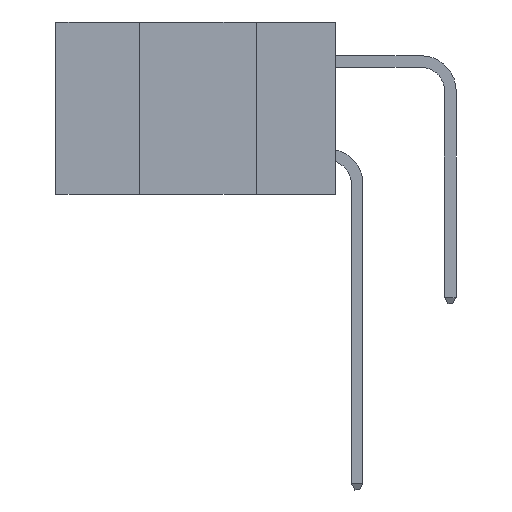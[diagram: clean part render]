
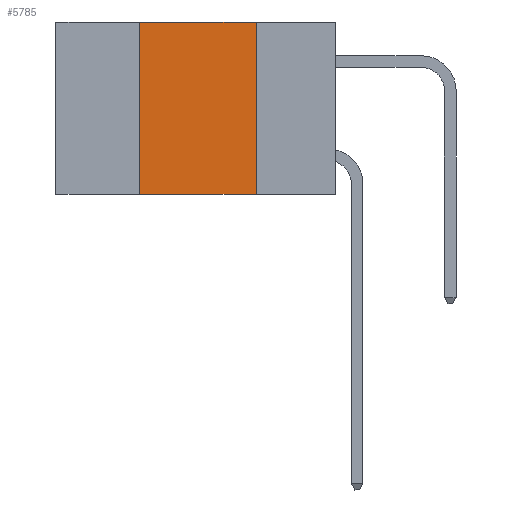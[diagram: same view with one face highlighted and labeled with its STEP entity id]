
A CAD part, left-side view. The second image highlights one B-rep face of the part: STEP entity #5785.
In plain terms, the highlighted planar face has unit normal (-1, 0, 0).
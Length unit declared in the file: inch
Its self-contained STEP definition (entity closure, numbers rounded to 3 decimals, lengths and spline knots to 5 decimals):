
#914 = VECTOR ( 'NONE', #7991, 39.37008 ) ;
#973 = CARTESIAN_POINT ( 'NONE',  ( 0., 0.6, -0.37 ) ) ;
#2066 = EDGE_CURVE ( 'NONE', #16141, #12509, #11155, .T. ) ;
#2370 = DIRECTION ( 'NONE',  ( 0., 0., -1. ) ) ;
#2549 = CARTESIAN_POINT ( 'NONE',  ( 0., 0.42, -0.37 ) ) ;
#2817 = CARTESIAN_POINT ( 'NONE',  ( 0., 0.6, 0. ) ) ;
#3033 = DIRECTION ( 'NONE',  ( 0., 0., 1. ) ) ;
#3947 = VECTOR ( 'NONE', #2370, 39.37008 ) ;
#4440 = LINE ( 'NONE', #2817, #914 ) ;
#5153 = EDGE_CURVE ( 'NONE', #16141, #13779, #15984, .T. ) ;
#5785 = ADVANCED_FACE ( 'NONE', ( #14710 ), #13887, .F. ) ;
#5922 = DIRECTION ( 'NONE',  ( 1., 0., 0. ) ) ;
#7413 = EDGE_CURVE ( 'NONE', #13779, #10472, #4440, .T. ) ;
#7991 = DIRECTION ( 'NONE',  ( 0., -1., 0. ) ) ;
#8312 = CARTESIAN_POINT ( 'NONE',  ( 0., 0.42, 0. ) ) ;
#8379 = ORIENTED_EDGE ( 'NONE', *, *, #7413, .F. ) ;
#8409 = DIRECTION ( 'NONE',  ( 0., 0., -1. ) ) ;
#8429 = CARTESIAN_POINT ( 'NONE',  ( 0., 0.42, 0. ) ) ;
#8545 = EDGE_LOOP ( 'NONE', ( #11046, #8379, #15216, #11092 ) ) ;
#9972 = AXIS2_PLACEMENT_3D ( 'NONE', #16394, #5922, #8409 ) ;
#10322 = CARTESIAN_POINT ( 'NONE',  ( 0., 0.17, 0. ) ) ;
#10472 = VERTEX_POINT ( 'NONE', #11791 ) ;
#11046 = ORIENTED_EDGE ( 'NONE', *, *, #14585, .F. ) ;
#11092 = ORIENTED_EDGE ( 'NONE', *, *, #2066, .T. ) ;
#11155 = LINE ( 'NONE', #973, #12201 ) ;
#11791 = CARTESIAN_POINT ( 'NONE',  ( 0., 0.17, 0. ) ) ;
#12201 = VECTOR ( 'NONE', #14175, 39.37008 ) ;
#12458 = CARTESIAN_POINT ( 'NONE',  ( 0., 0.17, -0.37 ) ) ;
#12509 = VERTEX_POINT ( 'NONE', #12458 ) ;
#12636 = VECTOR ( 'NONE', #3033, 39.37008 ) ;
#13543 = LINE ( 'NONE', #10322, #3947 ) ;
#13779 = VERTEX_POINT ( 'NONE', #8312 ) ;
#13887 = PLANE ( 'NONE',  #9972 ) ;
#14175 = DIRECTION ( 'NONE',  ( 0., -1., 0. ) ) ;
#14585 = EDGE_CURVE ( 'NONE', #10472, #12509, #13543, .T. ) ;
#14710 = FACE_OUTER_BOUND ( 'NONE', #8545, .T. ) ;
#15216 = ORIENTED_EDGE ( 'NONE', *, *, #5153, .F. ) ;
#15984 = LINE ( 'NONE', #8429, #12636 ) ;
#16141 = VERTEX_POINT ( 'NONE', #2549 ) ;
#16394 = CARTESIAN_POINT ( 'NONE',  ( 0., 0.6, 0. ) ) ;
